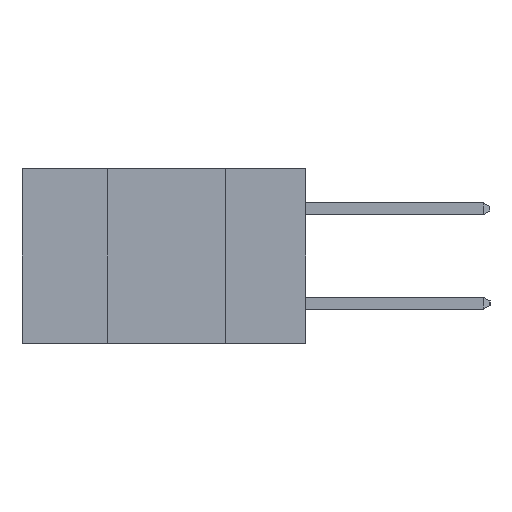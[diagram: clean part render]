
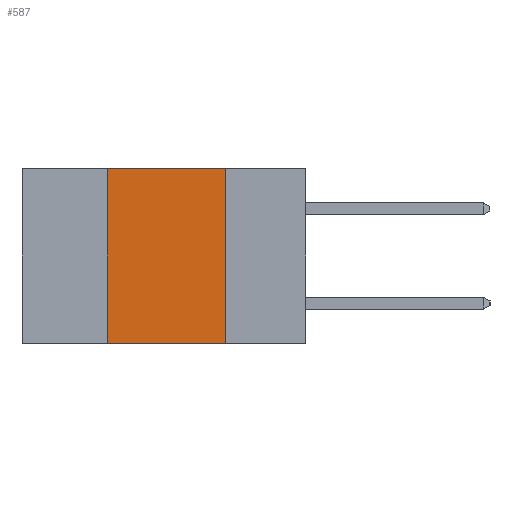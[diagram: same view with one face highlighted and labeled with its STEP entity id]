
A CAD part, left-side view. The second image highlights one B-rep face of the part: STEP entity #587.
In plain terms, the highlighted planar face has unit normal (-1, 0, 0).
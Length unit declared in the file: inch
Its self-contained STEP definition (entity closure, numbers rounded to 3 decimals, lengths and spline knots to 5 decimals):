
#101 = VECTOR ( 'NONE', #22393, 39.37008 ) ;
#587 = ADVANCED_FACE ( 'NONE', ( #11665 ), #25705, .F. ) ;
#3221 = LINE ( 'NONE', #10560, #8171 ) ;
#4408 = VERTEX_POINT ( 'NONE', #16897 ) ;
#5697 = LINE ( 'NONE', #8270, #101 ) ;
#5956 = ORIENTED_EDGE ( 'NONE', *, *, #19783, .F. ) ;
#6604 = ORIENTED_EDGE ( 'NONE', *, *, #11252, .F. ) ;
#7278 = ORIENTED_EDGE ( 'NONE', *, *, #23674, .F. ) ;
#7418 = CARTESIAN_POINT ( 'NONE',  ( 0., 0.17, 0. ) ) ;
#8171 = VECTOR ( 'NONE', #12612, 39.37008 ) ;
#8270 = CARTESIAN_POINT ( 'NONE',  ( 0., 0.6, 0. ) ) ;
#8383 = DIRECTION ( 'NONE',  ( 0., 0., 1. ) ) ;
#8484 = AXIS2_PLACEMENT_3D ( 'NONE', #25698, #24896, #20974 ) ;
#9622 = VECTOR ( 'NONE', #8383, 39.37008 ) ;
#10049 = EDGE_CURVE ( 'NONE', #4408, #10467, #14065, .T. ) ;
#10467 = VERTEX_POINT ( 'NONE', #23800 ) ;
#10560 = CARTESIAN_POINT ( 'NONE',  ( 0., 0.17, -0.37 ) ) ;
#11252 = EDGE_CURVE ( 'NONE', #16924, #22212, #5697, .T. ) ;
#11665 = FACE_OUTER_BOUND ( 'NONE', #16301, .T. ) ;
#12612 = DIRECTION ( 'NONE',  ( 0., 0., -1. ) ) ;
#14065 = LINE ( 'NONE', #14613, #18084 ) ;
#14613 = CARTESIAN_POINT ( 'NONE',  ( 0., 0.6, -0.37 ) ) ;
#16301 = EDGE_LOOP ( 'NONE', ( #7278, #6604, #5956, #25663 ) ) ;
#16897 = CARTESIAN_POINT ( 'NONE',  ( 0., 0.42, -0.37 ) ) ;
#16924 = VERTEX_POINT ( 'NONE', #17042 ) ;
#17042 = CARTESIAN_POINT ( 'NONE',  ( 0., 0.42, 0. ) ) ;
#18084 = VECTOR ( 'NONE', #18496, 39.37008 ) ;
#18496 = DIRECTION ( 'NONE',  ( 0., -1., 0. ) ) ;
#19783 = EDGE_CURVE ( 'NONE', #4408, #16924, #20139, .T. ) ;
#20139 = LINE ( 'NONE', #24219, #9622 ) ;
#20974 = DIRECTION ( 'NONE',  ( 0., 0., -1. ) ) ;
#22212 = VERTEX_POINT ( 'NONE', #7418 ) ;
#22393 = DIRECTION ( 'NONE',  ( 0., -1., 0. ) ) ;
#23674 = EDGE_CURVE ( 'NONE', #22212, #10467, #3221, .T. ) ;
#23800 = CARTESIAN_POINT ( 'NONE',  ( 0., 0.17, -0.37 ) ) ;
#24219 = CARTESIAN_POINT ( 'NONE',  ( 0., 0.42, -0.37 ) ) ;
#24896 = DIRECTION ( 'NONE',  ( 1., 0., 0. ) ) ;
#25663 = ORIENTED_EDGE ( 'NONE', *, *, #10049, .T. ) ;
#25698 = CARTESIAN_POINT ( 'NONE',  ( 0., 0.6, 0. ) ) ;
#25705 = PLANE ( 'NONE',  #8484 ) ;
